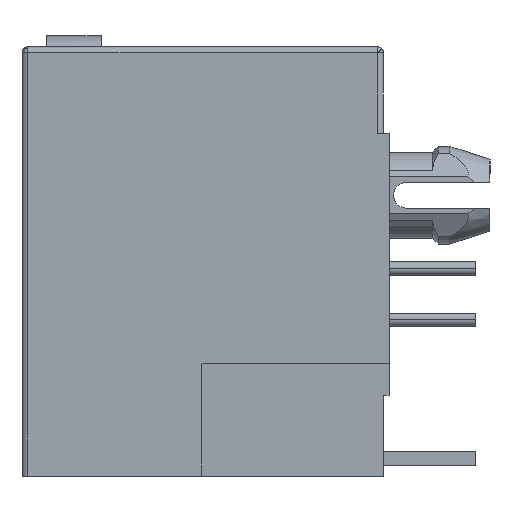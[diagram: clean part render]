
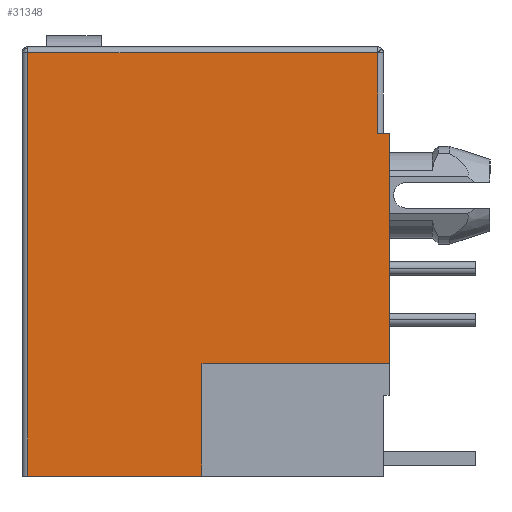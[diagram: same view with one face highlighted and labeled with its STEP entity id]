
A CAD part, left-side view. The second image highlights one B-rep face of the part: STEP entity #31348.
In plain terms, the highlighted planar face has unit normal (-1, 0, 0).
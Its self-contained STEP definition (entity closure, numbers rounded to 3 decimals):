
#12 = DIRECTION ( 'NONE',  ( 0., -1., 0. ) ) ;
#881 = EDGE_CURVE ( 'NONE', #46294, #7911, #29363, .T. ) ;
#1262 = VERTEX_POINT ( 'NONE', #39394 ) ;
#1748 = CARTESIAN_POINT ( 'NONE',  ( -8.025, -6.225, 7.325 ) ) ;
#3702 = CARTESIAN_POINT ( 'NONE',  ( -8.025, 0., 7.325 ) ) ;
#4687 = EDGE_CURVE ( 'NONE', #33718, #1262, #22303, .T. ) ;
#5163 = VECTOR ( 'NONE', #12, 1000. ) ;
#5568 = VECTOR ( 'NONE', #60589, 1000. ) ;
#6863 = DIRECTION ( 'NONE',  ( 0., 0., 1. ) ) ;
#7911 = VERTEX_POINT ( 'NONE', #33975 ) ;
#8884 = DIRECTION ( 'NONE',  ( 0., 1., 0. ) ) ;
#8981 = VECTOR ( 'NONE', #47634, 1000. ) ;
#9887 = ORIENTED_EDGE ( 'NONE', *, *, #4687, .T. ) ;
#11103 = VECTOR ( 'NONE', #6863, 1000. ) ;
#11580 = EDGE_CURVE ( 'NONE', #32269, #13473, #30284, .T. ) ;
#11718 = CARTESIAN_POINT ( 'NONE',  ( -8.025, -0.125, -3.475 ) ) ;
#13473 = VERTEX_POINT ( 'NONE', #22533 ) ;
#14675 = CARTESIAN_POINT ( 'NONE',  ( -8.025, 0., -3.475 ) ) ;
#15042 = CARTESIAN_POINT ( 'NONE',  ( -8.025, -6.625, 0. ) ) ;
#15642 = ORIENTED_EDGE ( 'NONE', *, *, #18008, .T. ) ;
#16195 = LINE ( 'NONE', #56546, #19257 ) ;
#16743 = ORIENTED_EDGE ( 'NONE', *, *, #57305, .F. ) ;
#18008 = EDGE_CURVE ( 'NONE', #61581, #46294, #21830, .T. ) ;
#19257 = VECTOR ( 'NONE', #8884, 1000. ) ;
#20838 = AXIS2_PLACEMENT_3D ( 'NONE', #53605, #24779, #29628 ) ;
#21171 = EDGE_CURVE ( 'NONE', #24268, #32269, #23381, .T. ) ;
#21555 = CARTESIAN_POINT ( 'NONE',  ( -8.025, -6.225, 4.525 ) ) ;
#21810 = ORIENTED_EDGE ( 'NONE', *, *, #881, .T. ) ;
#21830 = LINE ( 'NONE', #14675, #5163 ) ;
#22303 = LINE ( 'NONE', #22472, #5568 ) ;
#22461 = ORIENTED_EDGE ( 'NONE', *, *, #49722, .T. ) ;
#22472 = CARTESIAN_POINT ( 'NONE',  ( -8.025, 0., -7.375 ) ) ;
#22533 = CARTESIAN_POINT ( 'NONE',  ( -8.025, 5.925, 7.325 ) ) ;
#23381 = LINE ( 'NONE', #28657, #60256 ) ;
#24268 = VERTEX_POINT ( 'NONE', #21555 ) ;
#24779 = DIRECTION ( 'NONE',  ( -1., 0., 0. ) ) ;
#27666 = DIRECTION ( 'NONE',  ( 0., 1., 0. ) ) ;
#28657 = CARTESIAN_POINT ( 'NONE',  ( -8.025, -6.225, 0. ) ) ;
#29363 = LINE ( 'NONE', #15042, #8981 ) ;
#29575 = VECTOR ( 'NONE', #27666, 1000. ) ;
#29628 = DIRECTION ( 'NONE',  ( 0., -1., 0. ) ) ;
#29740 = CARTESIAN_POINT ( 'NONE',  ( -8.025, -0.125, 0. ) ) ;
#30284 = LINE ( 'NONE', #3702, #29575 ) ;
#30863 = ORIENTED_EDGE ( 'NONE', *, *, #46936, .T. ) ;
#30887 = VECTOR ( 'NONE', #58950, 1000. ) ;
#31348 = ADVANCED_FACE ( 'NONE', ( #36954 ), #39082, .T. ) ;
#32269 = VERTEX_POINT ( 'NONE', #1748 ) ;
#33718 = VERTEX_POINT ( 'NONE', #45776 ) ;
#33975 = CARTESIAN_POINT ( 'NONE',  ( -8.025, -6.625, 4.525 ) ) ;
#35264 = LINE ( 'NONE', #36448, #11103 ) ;
#36448 = CARTESIAN_POINT ( 'NONE',  ( -8.025, 5.925, 26.949 ) ) ;
#36954 = FACE_OUTER_BOUND ( 'NONE', #37383, .T. ) ;
#37383 = EDGE_LOOP ( 'NONE', ( #30863, #15642, #21810, #22461, #46579, #41801, #16743, #9887 ) ) ;
#38847 = CARTESIAN_POINT ( 'NONE',  ( -8.025, -6.625, -3.475 ) ) ;
#39082 = PLANE ( 'NONE',  #20838 ) ;
#39394 = CARTESIAN_POINT ( 'NONE',  ( -8.025, -0.125, -7.375 ) ) ;
#41801 = ORIENTED_EDGE ( 'NONE', *, *, #11580, .T. ) ;
#45776 = CARTESIAN_POINT ( 'NONE',  ( -8.025, 5.925, -7.375 ) ) ;
#46294 = VERTEX_POINT ( 'NONE', #38847 ) ;
#46579 = ORIENTED_EDGE ( 'NONE', *, *, #21171, .T. ) ;
#46936 = EDGE_CURVE ( 'NONE', #1262, #61581, #57246, .T. ) ;
#47634 = DIRECTION ( 'NONE',  ( 0., 0., 1. ) ) ;
#49722 = EDGE_CURVE ( 'NONE', #7911, #24268, #16195, .T. ) ;
#53605 = CARTESIAN_POINT ( 'NONE',  ( -8.025, 0., 0. ) ) ;
#56546 = CARTESIAN_POINT ( 'NONE',  ( -8.025, -6.635, 4.525 ) ) ;
#57246 = LINE ( 'NONE', #29740, #30887 ) ;
#57305 = EDGE_CURVE ( 'NONE', #33718, #13473, #35264, .T. ) ;
#58896 = DIRECTION ( 'NONE',  ( 0., 0., 1. ) ) ;
#58950 = DIRECTION ( 'NONE',  ( 0., 0., 1. ) ) ;
#60256 = VECTOR ( 'NONE', #58896, 1000. ) ;
#60589 = DIRECTION ( 'NONE',  ( 0., -1., 0. ) ) ;
#61581 = VERTEX_POINT ( 'NONE', #11718 ) ;
